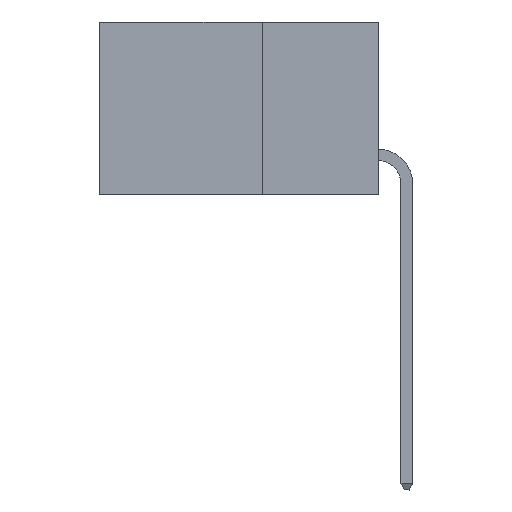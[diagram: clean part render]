
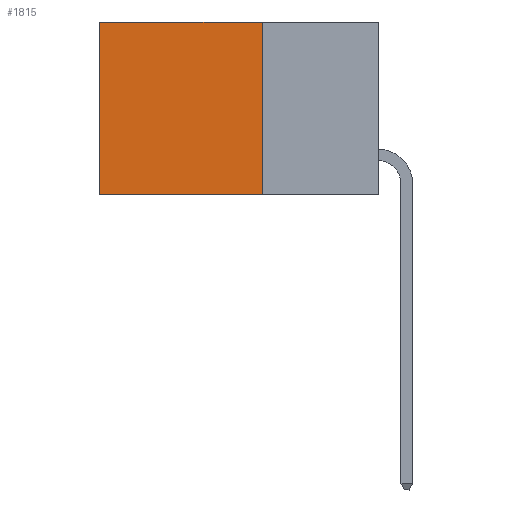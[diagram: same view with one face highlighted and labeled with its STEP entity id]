
A CAD part, left-side view. The second image highlights one B-rep face of the part: STEP entity #1815.
In plain terms, the highlighted planar face has unit normal (-1, 0, 0).
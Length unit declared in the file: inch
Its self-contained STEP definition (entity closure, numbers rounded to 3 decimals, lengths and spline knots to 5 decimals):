
#81 = EDGE_CURVE ( 'NONE', #593, #8114, #2019, .T. ) ;
#593 = VERTEX_POINT ( 'NONE', #5924 ) ;
#1182 = DIRECTION ( 'NONE',  ( 0., 0., -1. ) ) ;
#1221 = LINE ( 'NONE', #1565, #5032 ) ;
#1565 = CARTESIAN_POINT ( 'NONE',  ( 0.298, 0.25, 0. ) ) ;
#1815 = ADVANCED_FACE ( 'NONE', ( #7240 ), #7711, .F. ) ;
#2019 = LINE ( 'NONE', #8802, #7838 ) ;
#2451 = DIRECTION ( 'NONE',  ( 0., 0., -1. ) ) ;
#2693 = EDGE_CURVE ( 'NONE', #6873, #593, #4654, .T. ) ;
#3523 = CARTESIAN_POINT ( 'NONE',  ( 0.298, 0.25, 0. ) ) ;
#3706 = DIRECTION ( 'NONE',  ( 0., 1., 0. ) ) ;
#3854 = DIRECTION ( 'NONE',  ( 0., 1., 0. ) ) ;
#4053 = DIRECTION ( 'NONE',  ( 1., 0., 0. ) ) ;
#4114 = VERTEX_POINT ( 'NONE', #8373 ) ;
#4124 = DIRECTION ( 'NONE',  ( 0., 0., -1. ) ) ;
#4459 = EDGE_LOOP ( 'NONE', ( #9095, #6128, #8527, #5996 ) ) ;
#4552 = EDGE_CURVE ( 'NONE', #4114, #8114, #9016, .T. ) ;
#4612 = CARTESIAN_POINT ( 'NONE',  ( 0.298, 0.25, 0. ) ) ;
#4654 = LINE ( 'NONE', #3523, #4873 ) ;
#4805 = CARTESIAN_POINT ( 'NONE',  ( 0.298, 0.25, 0. ) ) ;
#4868 = VECTOR ( 'NONE', #1182, 39.37008 ) ;
#4873 = VECTOR ( 'NONE', #2451, 39.37008 ) ;
#5032 = VECTOR ( 'NONE', #3706, 39.37008 ) ;
#5110 = AXIS2_PLACEMENT_3D ( 'NONE', #4805, #4053, #4124 ) ;
#5924 = CARTESIAN_POINT ( 'NONE',  ( 0.298, 0.25, -0.37 ) ) ;
#5996 = ORIENTED_EDGE ( 'NONE', *, *, #8332, .T. ) ;
#6128 = ORIENTED_EDGE ( 'NONE', *, *, #81, .F. ) ;
#6873 = VERTEX_POINT ( 'NONE', #4612 ) ;
#7240 = FACE_OUTER_BOUND ( 'NONE', #4459, .T. ) ;
#7313 = CARTESIAN_POINT ( 'NONE',  ( 0.298, 0.6, -0.37 ) ) ;
#7521 = CARTESIAN_POINT ( 'NONE',  ( 0.298, 0.6, 0. ) ) ;
#7711 = PLANE ( 'NONE',  #5110 ) ;
#7838 = VECTOR ( 'NONE', #3854, 39.37008 ) ;
#8114 = VERTEX_POINT ( 'NONE', #7313 ) ;
#8332 = EDGE_CURVE ( 'NONE', #6873, #4114, #1221, .T. ) ;
#8373 = CARTESIAN_POINT ( 'NONE',  ( 0.298, 0.6, 0. ) ) ;
#8527 = ORIENTED_EDGE ( 'NONE', *, *, #2693, .F. ) ;
#8802 = CARTESIAN_POINT ( 'NONE',  ( 0.298, 0.25, -0.37 ) ) ;
#9016 = LINE ( 'NONE', #7521, #4868 ) ;
#9095 = ORIENTED_EDGE ( 'NONE', *, *, #4552, .T. ) ;
